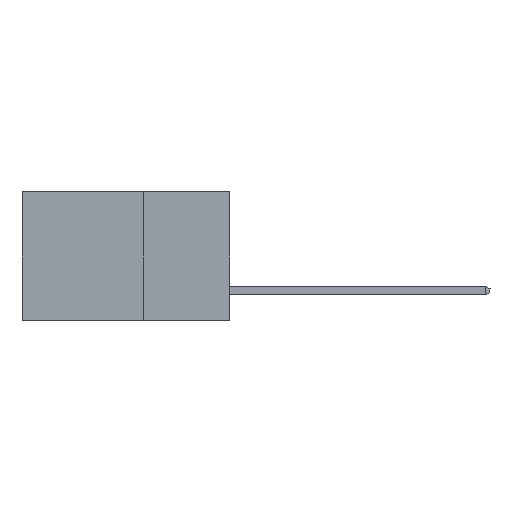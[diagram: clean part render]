
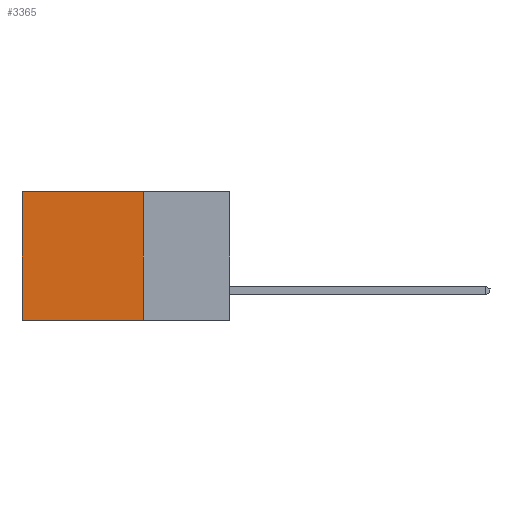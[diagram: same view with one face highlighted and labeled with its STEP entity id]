
A CAD part, left-side view. The second image highlights one B-rep face of the part: STEP entity #3365.
In plain terms, the highlighted planar face has unit normal (-1, 0, 0).
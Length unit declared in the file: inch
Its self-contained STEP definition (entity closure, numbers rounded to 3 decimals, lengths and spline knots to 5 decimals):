
#37 = VERTEX_POINT ( 'NONE', #3064 ) ;
#139 = ORIENTED_EDGE ( 'NONE', *, *, #3452, .F. ) ;
#461 = ORIENTED_EDGE ( 'NONE', *, *, #5924, .T. ) ;
#594 = PLANE ( 'NONE',  #8294 ) ;
#1212 = ORIENTED_EDGE ( 'NONE', *, *, #6873, .T. ) ;
#1454 = VECTOR ( 'NONE', #5515, 39.37008 ) ;
#1469 = CARTESIAN_POINT ( 'NONE',  ( 0.2615, 0.6, -0.37 ) ) ;
#1512 = VECTOR ( 'NONE', #3740, 39.37008 ) ;
#1989 = VERTEX_POINT ( 'NONE', #5150 ) ;
#2080 = DIRECTION ( 'NONE',  ( 0., 0., -1. ) ) ;
#2235 = LINE ( 'NONE', #5260, #1512 ) ;
#2285 = CARTESIAN_POINT ( 'NONE',  ( 0.2615, 0.25, -0.37 ) ) ;
#2537 = VECTOR ( 'NONE', #6960, 39.37008 ) ;
#2984 = DIRECTION ( 'NONE',  ( 1., 0., 0. ) ) ;
#3064 = CARTESIAN_POINT ( 'NONE',  ( 0.2615, 0.25, -0.37 ) ) ;
#3365 = ADVANCED_FACE ( 'NONE', ( #9387 ), #594, .F. ) ;
#3452 = EDGE_CURVE ( 'NONE', #37, #6422, #5312, .T. ) ;
#3740 = DIRECTION ( 'NONE',  ( 0., 1., 0. ) ) ;
#3761 = EDGE_CURVE ( 'NONE', #1989, #37, #8445, .T. ) ;
#4315 = CARTESIAN_POINT ( 'NONE',  ( 0.2615, 0.6, 0. ) ) ;
#5150 = CARTESIAN_POINT ( 'NONE',  ( 0.2615, 0.25, 0. ) ) ;
#5260 = CARTESIAN_POINT ( 'NONE',  ( 0.2615, 0.25, 0. ) ) ;
#5295 = ORIENTED_EDGE ( 'NONE', *, *, #3761, .F. ) ;
#5312 = LINE ( 'NONE', #9435, #1454 ) ;
#5515 = DIRECTION ( 'NONE',  ( 0., 1., 0. ) ) ;
#5924 = EDGE_CURVE ( 'NONE', #1989, #6686, #2235, .T. ) ;
#6188 = DIRECTION ( 'NONE',  ( 0., 0., -1. ) ) ;
#6422 = VERTEX_POINT ( 'NONE', #6935 ) ;
#6458 = VECTOR ( 'NONE', #2080, 39.37008 ) ;
#6686 = VERTEX_POINT ( 'NONE', #4315 ) ;
#6873 = EDGE_CURVE ( 'NONE', #6686, #6422, #8623, .T. ) ;
#6935 = CARTESIAN_POINT ( 'NONE',  ( 0.2615, 0.6, -0.37 ) ) ;
#6960 = DIRECTION ( 'NONE',  ( 0., 0., -1. ) ) ;
#8294 = AXIS2_PLACEMENT_3D ( 'NONE', #2285, #2984, #6188 ) ;
#8445 = LINE ( 'NONE', #8502, #6458 ) ;
#8502 = CARTESIAN_POINT ( 'NONE',  ( 0.2615, 0.25, -0.37 ) ) ;
#8623 = LINE ( 'NONE', #1469, #2537 ) ;
#9168 = EDGE_LOOP ( 'NONE', ( #1212, #139, #5295, #461 ) ) ;
#9387 = FACE_OUTER_BOUND ( 'NONE', #9168, .T. ) ;
#9435 = CARTESIAN_POINT ( 'NONE',  ( 0.2615, 0.25, -0.37 ) ) ;
